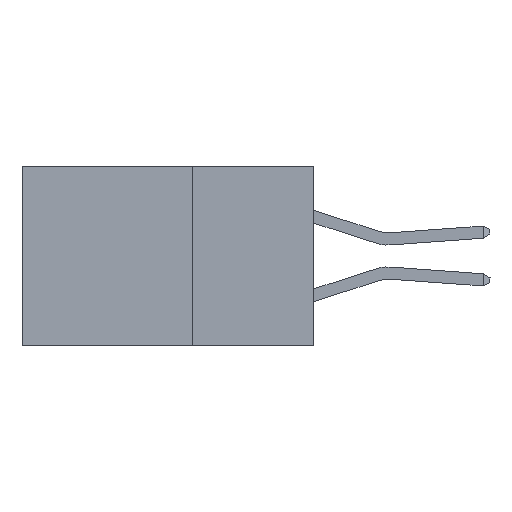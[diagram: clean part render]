
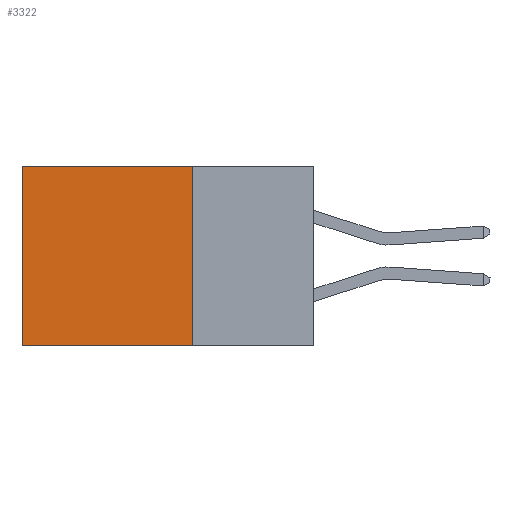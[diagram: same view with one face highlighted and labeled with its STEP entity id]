
A CAD part, left-side view. The second image highlights one B-rep face of the part: STEP entity #3322.
In plain terms, the highlighted planar face has unit normal (-1, 0, 0).
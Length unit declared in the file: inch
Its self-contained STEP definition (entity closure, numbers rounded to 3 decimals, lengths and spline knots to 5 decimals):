
#508 = VERTEX_POINT ( 'NONE', #1707 ) ;
#1264 = EDGE_CURVE ( 'NONE', #25054, #508, #26120, .T. ) ;
#1707 = CARTESIAN_POINT ( 'NONE',  ( 0.2875, 0.6, -0.37 ) ) ;
#2020 = PLANE ( 'NONE',  #19762 ) ;
#3195 = LINE ( 'NONE', #16427, #18557 ) ;
#3322 = ADVANCED_FACE ( 'NONE', ( #14595 ), #2020, .F. ) ;
#3378 = DIRECTION ( 'NONE',  ( 0., 1., 0. ) ) ;
#3762 = VERTEX_POINT ( 'NONE', #13507 ) ;
#3923 = DIRECTION ( 'NONE',  ( 1., 0., 0. ) ) ;
#7879 = CARTESIAN_POINT ( 'NONE',  ( 0.2875, 0.25, 0. ) ) ;
#8827 = CARTESIAN_POINT ( 'NONE',  ( 0.2875, 0.6, 0. ) ) ;
#10261 = DIRECTION ( 'NONE',  ( 0., 0., -1. ) ) ;
#11827 = ORIENTED_EDGE ( 'NONE', *, *, #19141, .F. ) ;
#12105 = EDGE_CURVE ( 'NONE', #3762, #17293, #26119, .T. ) ;
#12348 = ORIENTED_EDGE ( 'NONE', *, *, #1264, .F. ) ;
#13507 = CARTESIAN_POINT ( 'NONE',  ( 0.2875, 0.25, 0. ) ) ;
#14392 = VECTOR ( 'NONE', #3378, 39.37008 ) ;
#14595 = FACE_OUTER_BOUND ( 'NONE', #21927, .T. ) ;
#16043 = CARTESIAN_POINT ( 'NONE',  ( 0.2875, 0.25, 0. ) ) ;
#16427 = CARTESIAN_POINT ( 'NONE',  ( 0.2875, 0.25, 0. ) ) ;
#16953 = LINE ( 'NONE', #20661, #22860 ) ;
#17280 = CARTESIAN_POINT ( 'NONE',  ( 0.2875, 0.25, -0.37 ) ) ;
#17293 = VERTEX_POINT ( 'NONE', #8827 ) ;
#17841 = EDGE_CURVE ( 'NONE', #17293, #508, #16953, .T. ) ;
#18557 = VECTOR ( 'NONE', #20596, 39.37008 ) ;
#19141 = EDGE_CURVE ( 'NONE', #3762, #25054, #3195, .T. ) ;
#19762 = AXIS2_PLACEMENT_3D ( 'NONE', #16043, #3923, #25400 ) ;
#20596 = DIRECTION ( 'NONE',  ( 0., 0., -1. ) ) ;
#20661 = CARTESIAN_POINT ( 'NONE',  ( 0.2875, 0.6, 0. ) ) ;
#21927 = EDGE_LOOP ( 'NONE', ( #22629, #12348, #11827, #23179 ) ) ;
#21966 = DIRECTION ( 'NONE',  ( 0., 1., 0. ) ) ;
#22629 = ORIENTED_EDGE ( 'NONE', *, *, #17841, .T. ) ;
#22860 = VECTOR ( 'NONE', #10261, 39.37008 ) ;
#23179 = ORIENTED_EDGE ( 'NONE', *, *, #12105, .T. ) ;
#24802 = VECTOR ( 'NONE', #21966, 39.37008 ) ;
#25054 = VERTEX_POINT ( 'NONE', #17280 ) ;
#25400 = DIRECTION ( 'NONE',  ( 0., 0., -1. ) ) ;
#26119 = LINE ( 'NONE', #7879, #14392 ) ;
#26120 = LINE ( 'NONE', #26273, #24802 ) ;
#26273 = CARTESIAN_POINT ( 'NONE',  ( 0.2875, 0.25, -0.37 ) ) ;
